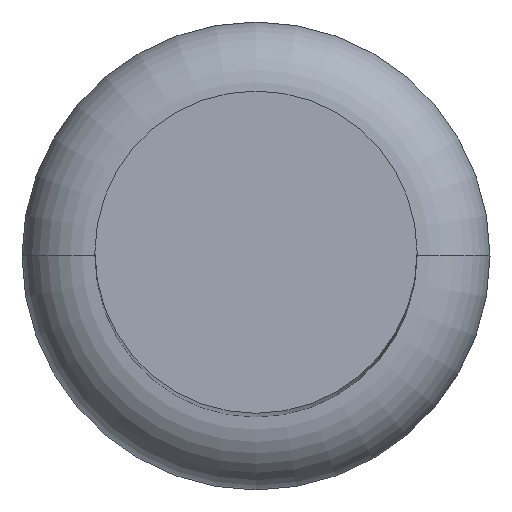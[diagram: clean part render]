
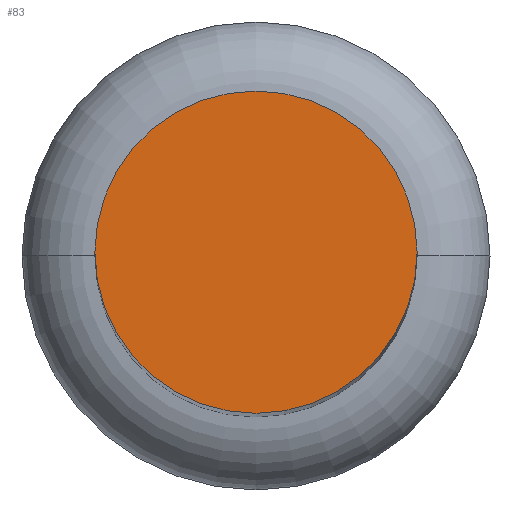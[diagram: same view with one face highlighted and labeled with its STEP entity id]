
A CAD part, top view. The second image highlights one B-rep face of the part: STEP entity #83.
In plain terms, the highlighted planar face has unit normal (0, 0, 1).
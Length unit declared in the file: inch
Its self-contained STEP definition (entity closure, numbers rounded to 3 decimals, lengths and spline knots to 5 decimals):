
#3 = CARTESIAN_POINT ( 'NONE',  ( 0., 0., 0. ) ) ;
#23 = AXIS2_PLACEMENT_3D ( 'NONE', #145, #160, #130 ) ;
#26 = DIRECTION ( 'NONE',  ( 1., 0., 0. ) ) ;
#28 = AXIS2_PLACEMENT_3D ( 'NONE', #121, #117, #26 ) ;
#36 = DIRECTION ( 'NONE',  ( 1., 0., 0. ) ) ;
#38 = EDGE_CURVE ( 'NONE', #173, #126, #77, .T. ) ;
#41 = PLANE ( 'NONE',  #176 ) ;
#43 = ORIENTED_EDGE ( 'NONE', *, *, #156, .T. ) ;
#46 = ORIENTED_EDGE ( 'NONE', *, *, #38, .T. ) ;
#77 = CIRCLE ( 'NONE', #23, 0.1 ) ;
#80 = EDGE_LOOP ( 'NONE', ( #43, #46 ) ) ;
#83 = ADVANCED_FACE ( 'NONE', ( #175 ), #41, .T. ) ;
#117 = DIRECTION ( 'NONE',  ( 0., 0., 1. ) ) ;
#121 = CARTESIAN_POINT ( 'NONE',  ( 0., 0., 0. ) ) ;
#126 = VERTEX_POINT ( 'NONE', #133 ) ;
#130 = DIRECTION ( 'NONE',  ( 1., 0., 0. ) ) ;
#132 = DIRECTION ( 'NONE',  ( 0., 0., 1. ) ) ;
#133 = CARTESIAN_POINT ( 'NONE',  ( 0.1, 0., 0. ) ) ;
#142 = CIRCLE ( 'NONE', #28, 0.1 ) ;
#145 = CARTESIAN_POINT ( 'NONE',  ( 0., 0., 0. ) ) ;
#156 = EDGE_CURVE ( 'NONE', #126, #173, #142, .T. ) ;
#160 = DIRECTION ( 'NONE',  ( 0., 0., 1. ) ) ;
#167 = CARTESIAN_POINT ( 'NONE',  ( -0.1, 0., 0. ) ) ;
#173 = VERTEX_POINT ( 'NONE', #167 ) ;
#175 = FACE_OUTER_BOUND ( 'NONE', #80, .T. ) ;
#176 = AXIS2_PLACEMENT_3D ( 'NONE', #3, #132, #36 ) ;
